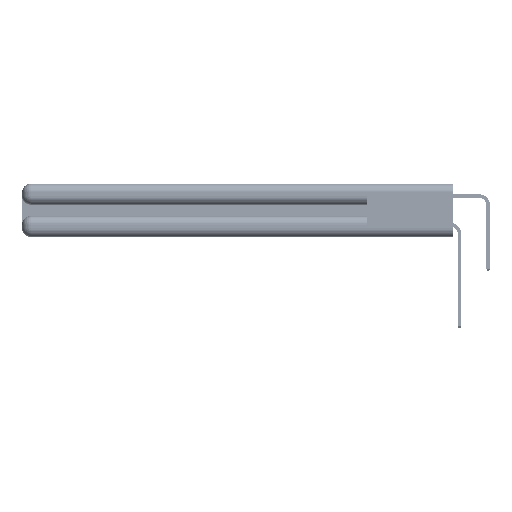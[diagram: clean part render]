
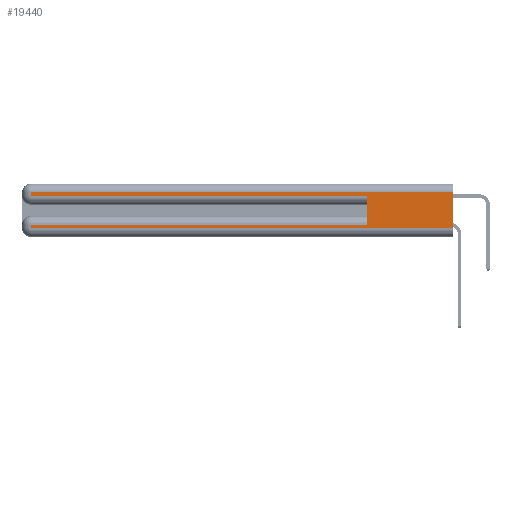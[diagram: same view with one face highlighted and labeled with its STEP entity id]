
A CAD part, left-side view. The second image highlights one B-rep face of the part: STEP entity #19440.
In plain terms, the highlighted planar face has unit normal (-1, 0, 0).
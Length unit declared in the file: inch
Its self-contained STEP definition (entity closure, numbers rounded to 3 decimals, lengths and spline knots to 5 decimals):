
#561 = EDGE_CURVE ( 'NONE', #31223, #24543, #9916, .T. ) ;
#1766 = VECTOR ( 'NONE', #48290, 39.37008 ) ;
#1854 = CARTESIAN_POINT ( 'NONE',  ( 0., 0., 0.06 ) ) ;
#2634 = DIRECTION ( 'NONE',  ( 0., 0., -1. ) ) ;
#3549 = VECTOR ( 'NONE', #3756, 39.37008 ) ;
#3615 = VERTEX_POINT ( 'NONE', #18892 ) ;
#3756 = DIRECTION ( 'NONE',  ( 0., 0., -1. ) ) ;
#5809 = CARTESIAN_POINT ( 'NONE',  ( 0., 0., 0.285 ) ) ;
#6955 = CARTESIAN_POINT ( 'NONE',  ( 0., 2.94, 0.31 ) ) ;
#7768 = CARTESIAN_POINT ( 'NONE',  ( 0., 0., 0.37 ) ) ;
#9236 = EDGE_CURVE ( 'NONE', #14558, #38511, #10018, .T. ) ;
#9287 = EDGE_LOOP ( 'NONE', ( #47388, #45608, #40078, #36543, #10322, #23420, #51733, #16398 ) ) ;
#9486 = CARTESIAN_POINT ( 'NONE',  ( 0., 2.94, 0.085 ) ) ;
#9916 = LINE ( 'NONE', #5809, #14418 ) ;
#10018 = LINE ( 'NONE', #44761, #3549 ) ;
#10244 = CARTESIAN_POINT ( 'NONE',  ( 0., 2.94, 0.06 ) ) ;
#10322 = ORIENTED_EDGE ( 'NONE', *, *, #10958, .F. ) ;
#10728 = EDGE_CURVE ( 'NONE', #24258, #35848, #24580, .T. ) ;
#10958 = EDGE_CURVE ( 'NONE', #3615, #24543, #32781, .T. ) ;
#14418 = VECTOR ( 'NONE', #19760, 39.37008 ) ;
#14558 = VERTEX_POINT ( 'NONE', #9486 ) ;
#15381 = PLANE ( 'NONE',  #21021 ) ;
#15718 = DIRECTION ( 'NONE',  ( 0., 0., -1. ) ) ;
#16398 = ORIENTED_EDGE ( 'NONE', *, *, #26554, .T. ) ;
#17475 = LINE ( 'NONE', #42143, #30821 ) ;
#17550 = FACE_OUTER_BOUND ( 'NONE', #9287, .T. ) ;
#17843 = DIRECTION ( 'NONE',  ( 0., 0., -1. ) ) ;
#18892 = CARTESIAN_POINT ( 'NONE',  ( 0., 0.6, 0.085 ) ) ;
#19320 = LINE ( 'NONE', #35699, #44739 ) ;
#19440 = ADVANCED_FACE ( 'NONE', ( #17550 ), #15381, .F. ) ;
#19760 = DIRECTION ( 'NONE',  ( 0., -1., 0. ) ) ;
#19898 = EDGE_CURVE ( 'NONE', #35848, #31223, #17475, .T. ) ;
#20682 = VECTOR ( 'NONE', #29890, 39.37008 ) ;
#21021 = AXIS2_PLACEMENT_3D ( 'NONE', #7768, #47893, #15718 ) ;
#23272 = CARTESIAN_POINT ( 'NONE',  ( 0., 0., 0.31 ) ) ;
#23420 = ORIENTED_EDGE ( 'NONE', *, *, #43477, .T. ) ;
#24258 = VERTEX_POINT ( 'NONE', #23272 ) ;
#24543 = VERTEX_POINT ( 'NONE', #51939 ) ;
#24580 = LINE ( 'NONE', #41625, #32174 ) ;
#25391 = CARTESIAN_POINT ( 'NONE',  ( 0., 0., 0.085 ) ) ;
#26554 = EDGE_CURVE ( 'NONE', #38511, #28210, #43108, .T. ) ;
#28210 = VERTEX_POINT ( 'NONE', #1854 ) ;
#29510 = DIRECTION ( 'NONE',  ( 0., -1., 0. ) ) ;
#29890 = DIRECTION ( 'NONE',  ( 0., 0., 1. ) ) ;
#30071 = DIRECTION ( 'NONE',  ( 0., 1., 0. ) ) ;
#30821 = VECTOR ( 'NONE', #17843, 39.37008 ) ;
#31223 = VERTEX_POINT ( 'NONE', #36015 ) ;
#32174 = VECTOR ( 'NONE', #30071, 39.37008 ) ;
#32781 = LINE ( 'NONE', #37881, #20682 ) ;
#35699 = CARTESIAN_POINT ( 'NONE',  ( 0., 0., 0.37 ) ) ;
#35848 = VERTEX_POINT ( 'NONE', #6955 ) ;
#36015 = CARTESIAN_POINT ( 'NONE',  ( 0., 2.94, 0.285 ) ) ;
#36543 = ORIENTED_EDGE ( 'NONE', *, *, #561, .T. ) ;
#37189 = EDGE_CURVE ( 'NONE', #24258, #28210, #19320, .T. ) ;
#37881 = CARTESIAN_POINT ( 'NONE',  ( 0., 0.6, 0.145 ) ) ;
#38511 = VERTEX_POINT ( 'NONE', #10244 ) ;
#38811 = LINE ( 'NONE', #25391, #1766 ) ;
#40078 = ORIENTED_EDGE ( 'NONE', *, *, #19898, .T. ) ;
#40727 = CARTESIAN_POINT ( 'NONE',  ( 0., 0., 0.06 ) ) ;
#41625 = CARTESIAN_POINT ( 'NONE',  ( 0., 0., 0.31 ) ) ;
#42143 = CARTESIAN_POINT ( 'NONE',  ( 0., 2.94, 0.37 ) ) ;
#43108 = LINE ( 'NONE', #40727, #45634 ) ;
#43477 = EDGE_CURVE ( 'NONE', #3615, #14558, #38811, .T. ) ;
#44739 = VECTOR ( 'NONE', #2634, 39.37008 ) ;
#44761 = CARTESIAN_POINT ( 'NONE',  ( 0., 2.94, 0.37 ) ) ;
#45608 = ORIENTED_EDGE ( 'NONE', *, *, #10728, .T. ) ;
#45634 = VECTOR ( 'NONE', #29510, 39.37008 ) ;
#47388 = ORIENTED_EDGE ( 'NONE', *, *, #37189, .F. ) ;
#47893 = DIRECTION ( 'NONE',  ( 1., 0., 0. ) ) ;
#48290 = DIRECTION ( 'NONE',  ( 0., 1., 0. ) ) ;
#51733 = ORIENTED_EDGE ( 'NONE', *, *, #9236, .T. ) ;
#51939 = CARTESIAN_POINT ( 'NONE',  ( 0., 0.6, 0.285 ) ) ;
